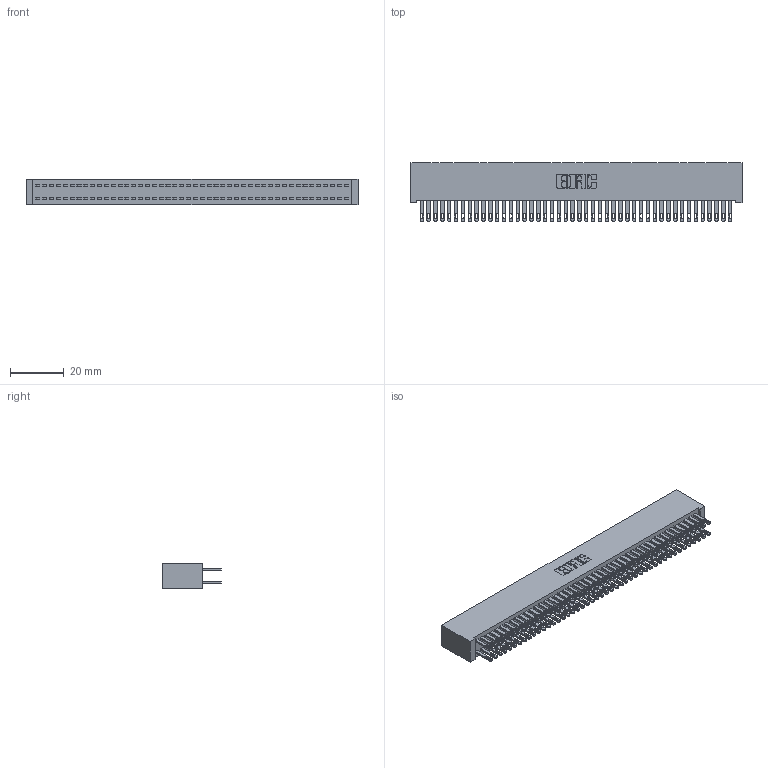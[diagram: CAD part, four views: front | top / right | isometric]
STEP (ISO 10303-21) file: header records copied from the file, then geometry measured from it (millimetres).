
FILE_DESCRIPTION (( 'STEP AP203' ), '1' );
FILE_NAME ('892-092-500-201.STEP', '2020-09-21T20:48:52', ( '' ), ( '' ), 'SwSTEP 2.0', 'SolidWorks 2020', '' );
FILE_SCHEMA (( 'CONFIG_CONTROL_DESIGN' ));
Length unit declared in the file: inch
Products named in the file (3): 892-092-500-201; 345-292-001_345-293-100; 842 Part_Lugless
Assembly tree (93 placements, depth 2):
  892-092-500-201
    842 Part_Lugless
    345-292-001_345-293-100  x92
Bounding box: 123.09 x 21.85 x 9.4 mm (x, y, z)
Volume: 11799.1 mm3; surface area: 20631.5 mm2
Topology: 93 solids, 93 shells, 4518 faces, 13799 edges, 9198 vertices
Faces by surface type: plane 2822, cylinder 1696
Entity records: 28597 total; most frequent: CARTESIAN_POINT 4730, ORIENTED_EDGE 4666, DIRECTION 4029, EDGE_CURVE 2333, VECTOR 2209, LINE 2209, VERTEX_POINT 1554, AXIS2_PLACEMENT_3D 910
